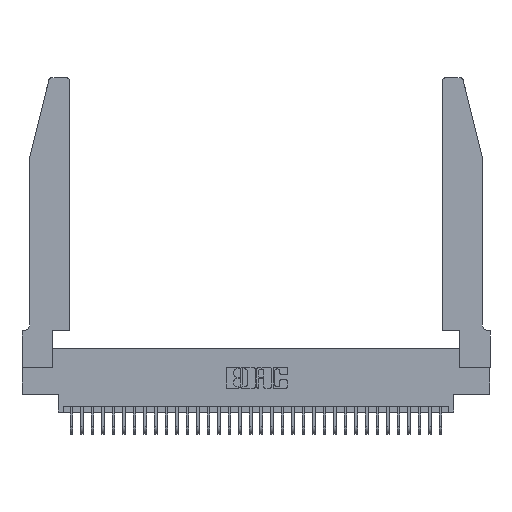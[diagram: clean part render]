
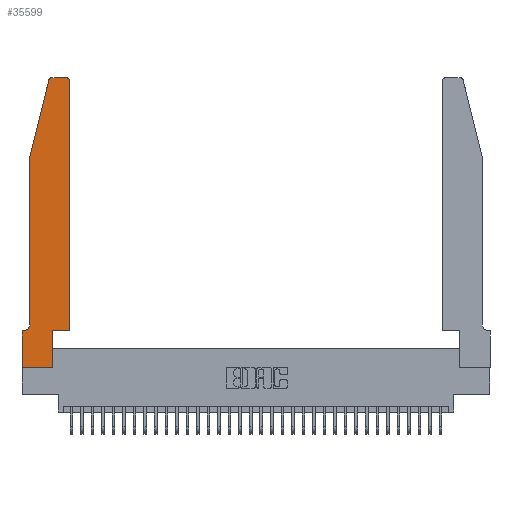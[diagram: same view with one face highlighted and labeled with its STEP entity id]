
A CAD part, top view. The second image highlights one B-rep face of the part: STEP entity #35599.
In plain terms, the highlighted planar face has unit normal (0, 0, 1).
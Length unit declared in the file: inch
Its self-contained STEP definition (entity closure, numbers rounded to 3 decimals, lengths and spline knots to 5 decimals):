
#878 = LINE ( 'NONE', #18058, #9224 ) ;
#1277 = EDGE_LOOP ( 'NONE', ( #9531, #5459, #35352, #34671, #2155, #3360, #13991, #34037, #21883, #35480, #29828, #24376 ) ) ;
#1330 = DIRECTION ( 'NONE',  ( 0., -1., 0. ) ) ;
#1413 = VERTEX_POINT ( 'NONE', #8702 ) ;
#1649 = VECTOR ( 'NONE', #7081, 39.37008 ) ;
#1658 = VERTEX_POINT ( 'NONE', #20817 ) ;
#1913 = DIRECTION ( 'NONE',  ( -1., 0., 0. ) ) ;
#2093 = DIRECTION ( 'NONE',  ( 1., 0., 0. ) ) ;
#2155 = ORIENTED_EDGE ( 'NONE', *, *, #25401, .T. ) ;
#2834 = VERTEX_POINT ( 'NONE', #20022 ) ;
#3098 = DIRECTION ( 'NONE',  ( 0., 0., 1. ) ) ;
#3265 = VECTOR ( 'NONE', #33895, 39.37008 ) ;
#3360 = ORIENTED_EDGE ( 'NONE', *, *, #29761, .T. ) ;
#3548 = EDGE_CURVE ( 'NONE', #2834, #5677, #28358, .T. ) ;
#4389 = EDGE_CURVE ( 'NONE', #32440, #1413, #10700, .T. ) ;
#4519 = VERTEX_POINT ( 'NONE', #26191 ) ;
#4714 = CARTESIAN_POINT ( 'NONE',  ( 0.0755, 0.35, 0.37 ) ) ;
#4773 = VERTEX_POINT ( 'NONE', #35270 ) ;
#5459 = ORIENTED_EDGE ( 'NONE', *, *, #19260, .T. ) ;
#5596 = CARTESIAN_POINT ( 'NONE',  ( 0.0755, 2., 0.37 ) ) ;
#5677 = VERTEX_POINT ( 'NONE', #28036 ) ;
#5772 = LINE ( 'NONE', #5596, #19677 ) ;
#6288 = LINE ( 'NONE', #4714, #34614 ) ;
#6580 = DIRECTION ( 'NONE',  ( 0., 0., 1. ) ) ;
#7081 = DIRECTION ( 'NONE',  ( 1., 0., 0. ) ) ;
#7878 = VECTOR ( 'NONE', #34497, 39.37008 ) ;
#8410 = DIRECTION ( 'NONE',  ( -0.239, -0.971, 0. ) ) ;
#8702 = CARTESIAN_POINT ( 'NONE',  ( 0.4505, 2.72, 0.37 ) ) ;
#9066 = EDGE_CURVE ( 'NONE', #30074, #34643, #20821, .T. ) ;
#9224 = VECTOR ( 'NONE', #1330, 39.37008 ) ;
#9325 = CARTESIAN_POINT ( 'NONE',  ( 0.0055, 0.42, 0.37 ) ) ;
#9531 = ORIENTED_EDGE ( 'NONE', *, *, #9066, .T. ) ;
#9559 = LINE ( 'NONE', #16160, #30576 ) ;
#9621 = CARTESIAN_POINT ( 'NONE',  ( 0.4505, 0.35, 0.37 ) ) ;
#10700 = LINE ( 'NONE', #28462, #3265 ) ;
#10806 = AXIS2_PLACEMENT_3D ( 'NONE', #30676, #14392, #33410 ) ;
#11009 = EDGE_CURVE ( 'NONE', #5677, #32440, #16523, .T. ) ;
#11432 = PLANE ( 'NONE',  #26380 ) ;
#11602 = CIRCLE ( 'NONE', #22545, 0.07 ) ;
#12165 = DIRECTION ( 'NONE',  ( -1., 0., 0. ) ) ;
#13257 = CARTESIAN_POINT ( 'NONE',  ( 0.2605, 2.75, 0.37 ) ) ;
#13513 = VECTOR ( 'NONE', #15921, 39.37008 ) ;
#13991 = ORIENTED_EDGE ( 'NONE', *, *, #31747, .T. ) ;
#14392 = DIRECTION ( 'NONE',  ( 0., 0., 1. ) ) ;
#15521 = CARTESIAN_POINT ( 'NONE',  ( 0.0755, 2., 0.37 ) ) ;
#15921 = DIRECTION ( 'NONE',  ( -1., 0., 0. ) ) ;
#16160 = CARTESIAN_POINT ( 'NONE',  ( 0., 0., 0.37 ) ) ;
#16213 = LINE ( 'NONE', #15521, #7878 ) ;
#16420 = FACE_OUTER_BOUND ( 'NONE', #1277, .T. ) ;
#16523 = LINE ( 'NONE', #18175, #1649 ) ;
#16588 = EDGE_CURVE ( 'NONE', #1658, #2834, #9559, .T. ) ;
#17505 = CARTESIAN_POINT ( 'NONE',  ( 0., 0.35, 0.37 ) ) ;
#18058 = CARTESIAN_POINT ( 'NONE',  ( 0., 0., 0.37 ) ) ;
#18175 = CARTESIAN_POINT ( 'NONE',  ( 0.4505, 0.35, 0.37 ) ) ;
#18448 = CIRCLE ( 'NONE', #22991, 0.03 ) ;
#19260 = EDGE_CURVE ( 'NONE', #34643, #4519, #33781, .T. ) ;
#19417 = VERTEX_POINT ( 'NONE', #23078 ) ;
#19677 = VECTOR ( 'NONE', #8410, 39.37008 ) ;
#19747 = CARTESIAN_POINT ( 'NONE',  ( 0., 0.35, 0.37 ) ) ;
#20022 = CARTESIAN_POINT ( 'NONE',  ( 0.2865, 0., 0.37 ) ) ;
#20320 = EDGE_CURVE ( 'NONE', #4519, #28410, #5772, .T. ) ;
#20817 = CARTESIAN_POINT ( 'NONE',  ( 0., 0., 0.37 ) ) ;
#20821 = LINE ( 'NONE', #13257, #13513 ) ;
#21143 = VECTOR ( 'NONE', #32992, 39.37008 ) ;
#21883 = ORIENTED_EDGE ( 'NONE', *, *, #3548, .T. ) ;
#22094 = EDGE_CURVE ( 'NONE', #28410, #4773, #16213, .T. ) ;
#22498 = DIRECTION ( 'NONE',  ( 1., 0., 0. ) ) ;
#22545 = AXIS2_PLACEMENT_3D ( 'NONE', #9325, #28533, #12165 ) ;
#22991 = AXIS2_PLACEMENT_3D ( 'NONE', #23144, #6580, #25868 ) ;
#23078 = CARTESIAN_POINT ( 'NONE',  ( 0.0055, 0.35, 0.37 ) ) ;
#23144 = CARTESIAN_POINT ( 'NONE',  ( 0.4205, 2.72, 0.37 ) ) ;
#24376 = ORIENTED_EDGE ( 'NONE', *, *, #26079, .T. ) ;
#25401 = EDGE_CURVE ( 'NONE', #4773, #19417, #11602, .T. ) ;
#25868 = DIRECTION ( 'NONE',  ( 1., 0., 0. ) ) ;
#26079 = EDGE_CURVE ( 'NONE', #1413, #30074, #18448, .T. ) ;
#26191 = CARTESIAN_POINT ( 'NONE',  ( 0.25487, 2.72718, 0.37 ) ) ;
#26380 = AXIS2_PLACEMENT_3D ( 'NONE', #19747, #3098, #22498 ) ;
#28036 = CARTESIAN_POINT ( 'NONE',  ( 0.2865, 0.35, 0.37 ) ) ;
#28358 = LINE ( 'NONE', #30267, #21143 ) ;
#28410 = VERTEX_POINT ( 'NONE', #32203 ) ;
#28462 = CARTESIAN_POINT ( 'NONE',  ( 0.4505, 0.35, 0.37 ) ) ;
#28533 = DIRECTION ( 'NONE',  ( 0., 0., -1. ) ) ;
#29761 = EDGE_CURVE ( 'NONE', #19417, #34904, #6288, .T. ) ;
#29828 = ORIENTED_EDGE ( 'NONE', *, *, #4389, .T. ) ;
#30074 = VERTEX_POINT ( 'NONE', #30994 ) ;
#30267 = CARTESIAN_POINT ( 'NONE',  ( 0.2865, 0.35, 0.37 ) ) ;
#30576 = VECTOR ( 'NONE', #2093, 39.37008 ) ;
#30676 = CARTESIAN_POINT ( 'NONE',  ( 0.284, 2.72, 0.37 ) ) ;
#30994 = CARTESIAN_POINT ( 'NONE',  ( 0.4205, 2.75, 0.37 ) ) ;
#31747 = EDGE_CURVE ( 'NONE', #34904, #1658, #878, .T. ) ;
#32203 = CARTESIAN_POINT ( 'NONE',  ( 0.0755, 2., 0.37 ) ) ;
#32365 = CARTESIAN_POINT ( 'NONE',  ( 0.284, 2.75, 0.37 ) ) ;
#32440 = VERTEX_POINT ( 'NONE', #9621 ) ;
#32992 = DIRECTION ( 'NONE',  ( 0., 1., 0. ) ) ;
#33410 = DIRECTION ( 'NONE',  ( 1., 0., 0. ) ) ;
#33781 = CIRCLE ( 'NONE', #10806, 0.03 ) ;
#33895 = DIRECTION ( 'NONE',  ( 0., 1., 0. ) ) ;
#34037 = ORIENTED_EDGE ( 'NONE', *, *, #16588, .T. ) ;
#34497 = DIRECTION ( 'NONE',  ( 0., -1., 0. ) ) ;
#34614 = VECTOR ( 'NONE', #1913, 39.37008 ) ;
#34643 = VERTEX_POINT ( 'NONE', #32365 ) ;
#34671 = ORIENTED_EDGE ( 'NONE', *, *, #22094, .T. ) ;
#34904 = VERTEX_POINT ( 'NONE', #17505 ) ;
#35270 = CARTESIAN_POINT ( 'NONE',  ( 0.0755, 0.42, 0.37 ) ) ;
#35352 = ORIENTED_EDGE ( 'NONE', *, *, #20320, .T. ) ;
#35480 = ORIENTED_EDGE ( 'NONE', *, *, #11009, .T. ) ;
#35599 = ADVANCED_FACE ( 'NONE', ( #16420 ), #11432, .T. ) ;
